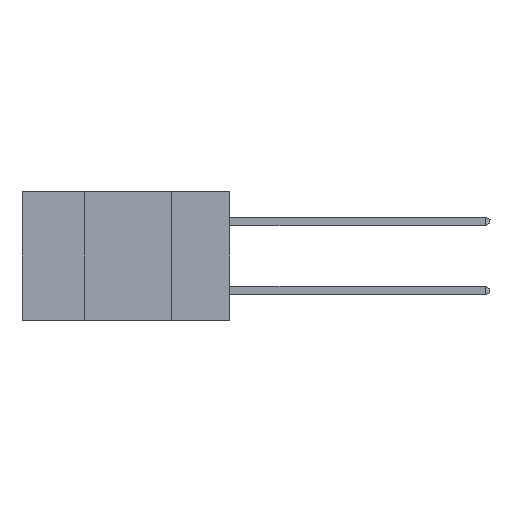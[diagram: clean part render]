
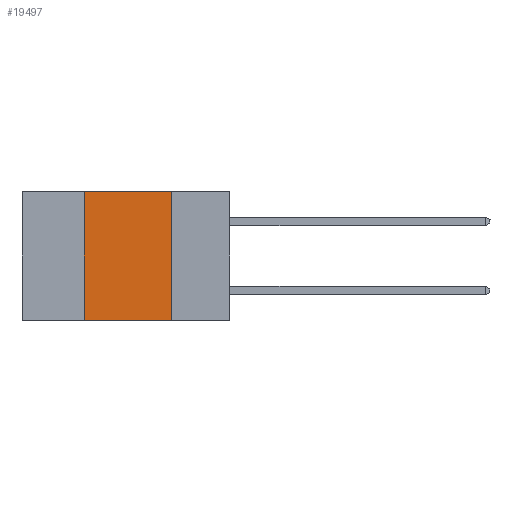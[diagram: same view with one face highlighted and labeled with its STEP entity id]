
A CAD part, left-side view. The second image highlights one B-rep face of the part: STEP entity #19497.
In plain terms, the highlighted planar face has unit normal (-1, 0, 0).
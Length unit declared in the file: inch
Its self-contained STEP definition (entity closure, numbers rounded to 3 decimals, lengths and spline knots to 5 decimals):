
#485 = CARTESIAN_POINT ( 'NONE',  ( 0., 0.6, 0. ) ) ;
#1277 = LINE ( 'NONE', #5376, #6761 ) ;
#1655 = ORIENTED_EDGE ( 'NONE', *, *, #7929, .F. ) ;
#2048 = VERTEX_POINT ( 'NONE', #8371 ) ;
#2412 = FACE_OUTER_BOUND ( 'NONE', #9272, .T. ) ;
#3396 = DIRECTION ( 'NONE',  ( 0., 0., -1. ) ) ;
#5376 = CARTESIAN_POINT ( 'NONE',  ( 0., 0.6, -0.37 ) ) ;
#5790 = DIRECTION ( 'NONE',  ( 1., 0., 0. ) ) ;
#5889 = CARTESIAN_POINT ( 'NONE',  ( 0., 0.6, 0. ) ) ;
#6604 = LINE ( 'NONE', #13984, #16370 ) ;
#6761 = VECTOR ( 'NONE', #21726, 39.37008 ) ;
#7472 = VECTOR ( 'NONE', #21027, 39.37008 ) ;
#7929 = EDGE_CURVE ( 'NONE', #18959, #2048, #17939, .T. ) ;
#8371 = CARTESIAN_POINT ( 'NONE',  ( 0., 0.17, -0.37 ) ) ;
#9065 = CARTESIAN_POINT ( 'NONE',  ( 0., 0.42, -0.37 ) ) ;
#9272 = EDGE_LOOP ( 'NONE', ( #1655, #22666, #9830, #17517 ) ) ;
#9830 = ORIENTED_EDGE ( 'NONE', *, *, #21614, .F. ) ;
#10909 = CARTESIAN_POINT ( 'NONE',  ( 0., 0.17, -0.37 ) ) ;
#11536 = AXIS2_PLACEMENT_3D ( 'NONE', #485, #5790, #20698 ) ;
#13319 = CARTESIAN_POINT ( 'NONE',  ( 0., 0.42, 0. ) ) ;
#13365 = VERTEX_POINT ( 'NONE', #9065 ) ;
#13984 = CARTESIAN_POINT ( 'NONE',  ( 0., 0.42, -0.37 ) ) ;
#15692 = EDGE_CURVE ( 'NONE', #13365, #2048, #1277, .T. ) ;
#16370 = VECTOR ( 'NONE', #17889, 39.37008 ) ;
#16893 = VERTEX_POINT ( 'NONE', #13319 ) ;
#17517 = ORIENTED_EDGE ( 'NONE', *, *, #15692, .T. ) ;
#17889 = DIRECTION ( 'NONE',  ( 0., 0., 1. ) ) ;
#17939 = LINE ( 'NONE', #10909, #19748 ) ;
#18959 = VERTEX_POINT ( 'NONE', #20473 ) ;
#19497 = ADVANCED_FACE ( 'NONE', ( #2412 ), #22395, .F. ) ;
#19748 = VECTOR ( 'NONE', #3396, 39.37008 ) ;
#20473 = CARTESIAN_POINT ( 'NONE',  ( 0., 0.17, 0. ) ) ;
#20698 = DIRECTION ( 'NONE',  ( 0., 0., -1. ) ) ;
#20907 = LINE ( 'NONE', #5889, #7472 ) ;
#21027 = DIRECTION ( 'NONE',  ( 0., -1., 0. ) ) ;
#21406 = EDGE_CURVE ( 'NONE', #16893, #18959, #20907, .T. ) ;
#21614 = EDGE_CURVE ( 'NONE', #13365, #16893, #6604, .T. ) ;
#21726 = DIRECTION ( 'NONE',  ( 0., -1., 0. ) ) ;
#22395 = PLANE ( 'NONE',  #11536 ) ;
#22666 = ORIENTED_EDGE ( 'NONE', *, *, #21406, .F. ) ;
